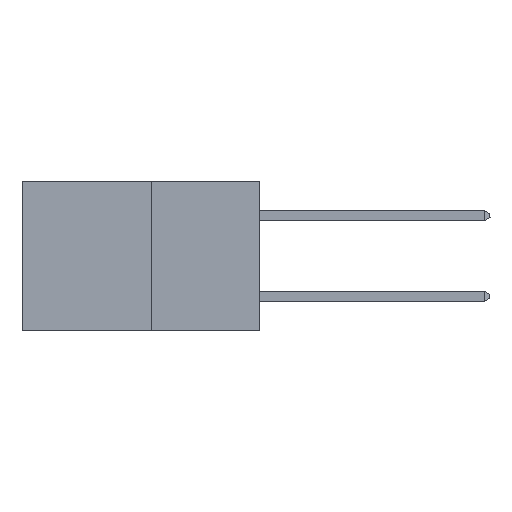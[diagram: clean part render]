
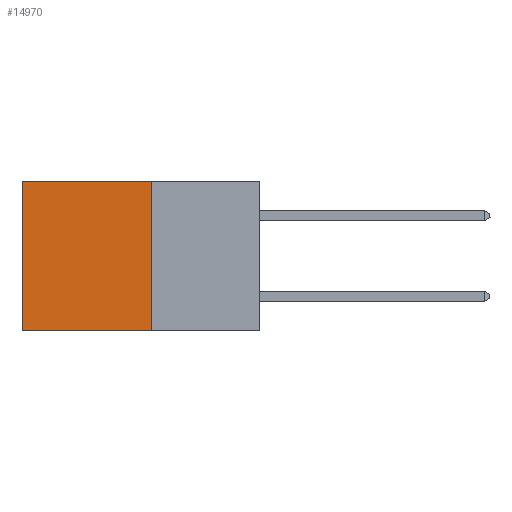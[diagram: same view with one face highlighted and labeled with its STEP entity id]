
A CAD part, left-side view. The second image highlights one B-rep face of the part: STEP entity #14970.
In plain terms, the highlighted planar face has unit normal (-1, 0, 0).
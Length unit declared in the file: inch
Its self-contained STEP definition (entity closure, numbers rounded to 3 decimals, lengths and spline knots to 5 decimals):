
#276 = DIRECTION ( 'NONE',  ( 0., 0., -1. ) ) ;
#1125 = ORIENTED_EDGE ( 'NONE', *, *, #12029, .F. ) ;
#1137 = EDGE_LOOP ( 'NONE', ( #15676, #1125, #2767, #7782 ) ) ;
#1833 = AXIS2_PLACEMENT_3D ( 'NONE', #7569, #8980, #276 ) ;
#2262 = FACE_OUTER_BOUND ( 'NONE', #1137, .T. ) ;
#2669 = DIRECTION ( 'NONE',  ( 0., 0., -1. ) ) ;
#2767 = ORIENTED_EDGE ( 'NONE', *, *, #4885, .F. ) ;
#2975 = CARTESIAN_POINT ( 'NONE',  ( 0.277, 0.59, 0. ) ) ;
#3092 = VECTOR ( 'NONE', #16611, 39.37008 ) ;
#4885 = EDGE_CURVE ( 'NONE', #5040, #7323, #5242, .T. ) ;
#5040 = VERTEX_POINT ( 'NONE', #16379 ) ;
#5242 = LINE ( 'NONE', #9694, #12783 ) ;
#5748 = LINE ( 'NONE', #17080, #12361 ) ;
#5854 = CARTESIAN_POINT ( 'NONE',  ( 0.277, 0.27, -0.37 ) ) ;
#6511 = CARTESIAN_POINT ( 'NONE',  ( 0.277, 0.27, -0.37 ) ) ;
#6979 = DIRECTION ( 'NONE',  ( 0., 1., 0. ) ) ;
#7323 = VERTEX_POINT ( 'NONE', #5854 ) ;
#7569 = CARTESIAN_POINT ( 'NONE',  ( 0.277, 0.27, -0.37 ) ) ;
#7577 = VERTEX_POINT ( 'NONE', #2975 ) ;
#7782 = ORIENTED_EDGE ( 'NONE', *, *, #12845, .T. ) ;
#8980 = DIRECTION ( 'NONE',  ( 1., 0., 0. ) ) ;
#9694 = CARTESIAN_POINT ( 'NONE',  ( 0.277, 0.27, -0.37 ) ) ;
#10289 = CARTESIAN_POINT ( 'NONE',  ( 0.277, 0.59, -0.37 ) ) ;
#11157 = EDGE_CURVE ( 'NONE', #7577, #14949, #5748, .T. ) ;
#11591 = LINE ( 'NONE', #6511, #3092 ) ;
#12029 = EDGE_CURVE ( 'NONE', #7323, #14949, #11591, .T. ) ;
#12361 = VECTOR ( 'NONE', #12623, 39.37008 ) ;
#12623 = DIRECTION ( 'NONE',  ( 0., 0., -1. ) ) ;
#12783 = VECTOR ( 'NONE', #2669, 39.37008 ) ;
#12845 = EDGE_CURVE ( 'NONE', #5040, #7577, #14121, .T. ) ;
#14121 = LINE ( 'NONE', #17024, #17543 ) ;
#14949 = VERTEX_POINT ( 'NONE', #10289 ) ;
#14970 = ADVANCED_FACE ( 'NONE', ( #2262 ), #17679, .F. ) ;
#15676 = ORIENTED_EDGE ( 'NONE', *, *, #11157, .T. ) ;
#16379 = CARTESIAN_POINT ( 'NONE',  ( 0.277, 0.27, 0. ) ) ;
#16611 = DIRECTION ( 'NONE',  ( 0., 1., 0. ) ) ;
#17024 = CARTESIAN_POINT ( 'NONE',  ( 0.277, 0.27, 0. ) ) ;
#17080 = CARTESIAN_POINT ( 'NONE',  ( 0.277, 0.59, -0.37 ) ) ;
#17543 = VECTOR ( 'NONE', #6979, 39.37008 ) ;
#17679 = PLANE ( 'NONE',  #1833 ) ;
